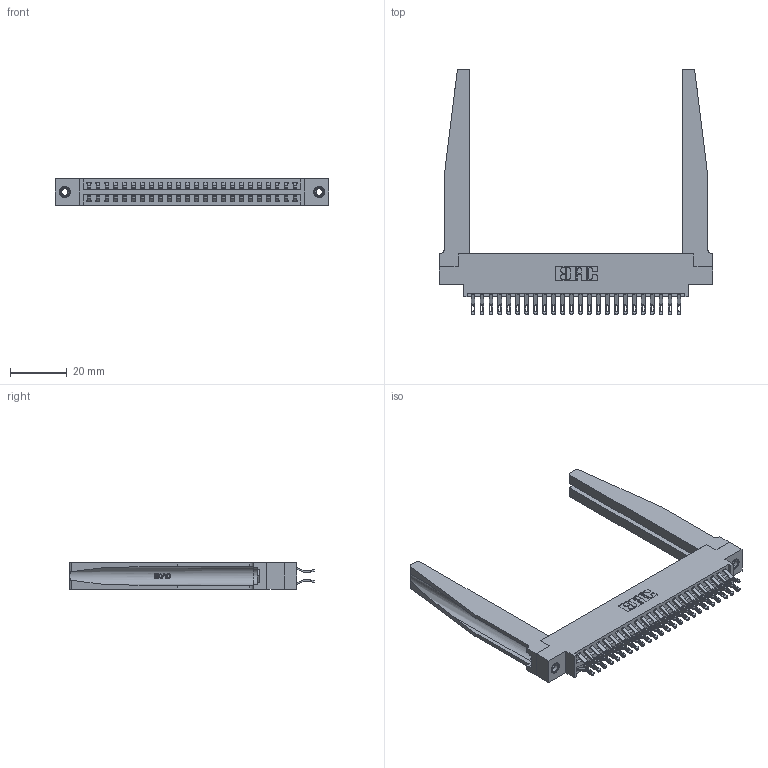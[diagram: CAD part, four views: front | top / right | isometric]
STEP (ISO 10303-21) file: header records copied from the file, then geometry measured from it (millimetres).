
FILE_DESCRIPTION (( 'STEP AP203' ), '1' );
FILE_NAME ('396-048-555-878.STEP', '2019-11-02T07:06:53', ( '' ), ( '' ), 'SwSTEP 2.0', 'SolidWorks 2016', '' );
FILE_SCHEMA (( 'CONFIG_CONTROL_DESIGN' ));
Length unit declared in the file: inch
Products named in the file (5): 346 Part_0.170 Offset - 0.156 Dia-TH; 345-292-001_555 Tail; 346-220-078_345-220-078; 345-250-001_345-250-001-102; 396-048-555-878
Assembly tree (53 placements, depth 2):
  396-048-555-878
    346 Part_0.170 Offset - 0.156 Dia-TH
    345-292-001_555 Tail  x48
    346-220-078_345-220-078  x2
    345-250-001_345-250-001-102  x2
Bounding box: 96.77 x 86.74 x 9.4 mm (x, y, z)
Volume: 16190.3 mm3; surface area: 19688.5 mm2
Topology: 53 solids, 53 shells, 3144 faces, 9733 edges, 6478 vertices
Faces by surface type: plane 1806, cylinder 1286, bspline 36, cone 12, torus 4
Entity records: 23292 total; most frequent: CARTESIAN_POINT 4837, ORIENTED_EDGE 3630, DIRECTION 3269, EDGE_CURVE 1815, VECTOR 1473, LINE 1473, VERTEX_POINT 1204, AXIS2_PLACEMENT_3D 898
